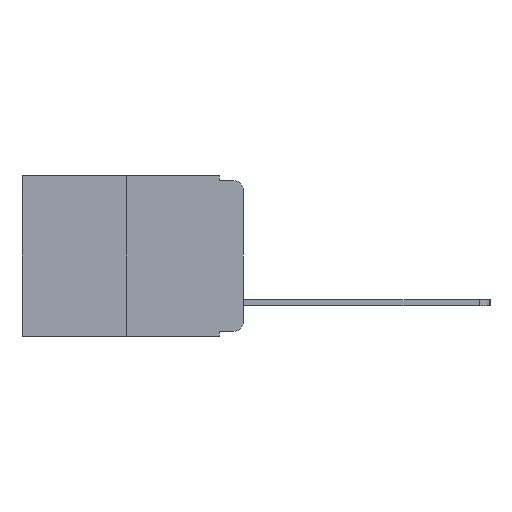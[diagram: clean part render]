
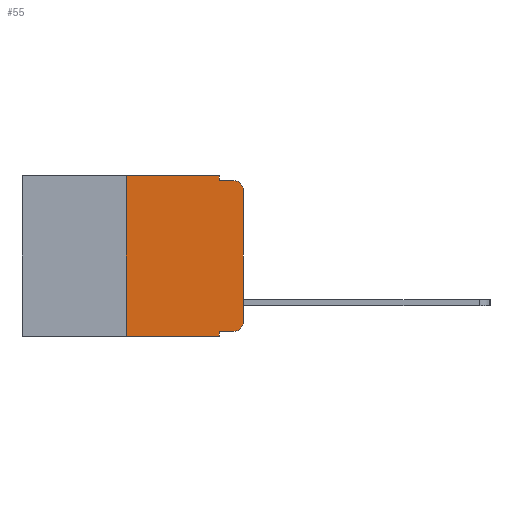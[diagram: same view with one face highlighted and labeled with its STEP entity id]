
A CAD part, left-side view. The second image highlights one B-rep face of the part: STEP entity #55.
In plain terms, the highlighted planar face has unit normal (-1, 0, 0).
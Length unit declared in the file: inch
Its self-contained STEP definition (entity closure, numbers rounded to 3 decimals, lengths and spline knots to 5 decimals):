
#55 = ADVANCED_FACE ( 'NONE', ( #7091 ), #18615, .F. ) ;
#433 = VECTOR ( 'NONE', #20147, 39.37008 ) ;
#586 = VECTOR ( 'NONE', #16774, 39.37008 ) ;
#597 = VERTEX_POINT ( 'NONE', #14116 ) ;
#598 = VERTEX_POINT ( 'NONE', #16816 ) ;
#1123 = ORIENTED_EDGE ( 'NONE', *, *, #10731, .F. ) ;
#1836 = EDGE_LOOP ( 'NONE', ( #14913, #14934, #15651, #18490, #20879, #17882, #7262, #1123, #14017, #13788 ) ) ;
#1862 = VERTEX_POINT ( 'NONE', #4529 ) ;
#2223 = DIRECTION ( 'NONE',  ( -1., 0., 0. ) ) ;
#2350 = CIRCLE ( 'NONE', #5053, 0.02 ) ;
#2389 = LINE ( 'NONE', #4756, #18641 ) ;
#2857 = DIRECTION ( 'NONE',  ( 1., 0., 0. ) ) ;
#3148 = VERTEX_POINT ( 'NONE', #18737 ) ;
#3492 = CARTESIAN_POINT ( 'NONE',  ( 0., 0.25, 0. ) ) ;
#3639 = VERTEX_POINT ( 'NONE', #6182 ) ;
#3965 = EDGE_CURVE ( 'NONE', #8774, #598, #14418, .T. ) ;
#4018 = DIRECTION ( 'NONE',  ( -1., 0., 0. ) ) ;
#4388 = EDGE_CURVE ( 'NONE', #3639, #8774, #10649, .T. ) ;
#4433 = LINE ( 'NONE', #15539, #433 ) ;
#4529 = CARTESIAN_POINT ( 'NONE',  ( 0., 0., -0.03 ) ) ;
#4756 = CARTESIAN_POINT ( 'NONE',  ( 0., 0.051, -0.333 ) ) ;
#5053 = AXIS2_PLACEMENT_3D ( 'NONE', #12225, #2223, #13810 ) ;
#5112 = DIRECTION ( 'NONE',  ( 0., 0., -1. ) ) ;
#5128 = LINE ( 'NONE', #10507, #586 ) ;
#5512 = DIRECTION ( 'NONE',  ( 0., -1., 0. ) ) ;
#5870 = AXIS2_PLACEMENT_3D ( 'NONE', #13924, #4018, #15485 ) ;
#6182 = CARTESIAN_POINT ( 'NONE',  ( 0., 0.051, 0. ) ) ;
#6420 = DIRECTION ( 'NONE',  ( 0., -1., 0. ) ) ;
#7091 = FACE_OUTER_BOUND ( 'NONE', #1836, .T. ) ;
#7262 = ORIENTED_EDGE ( 'NONE', *, *, #19911, .T. ) ;
#7589 = VECTOR ( 'NONE', #18061, 39.37008 ) ;
#7633 = VERTEX_POINT ( 'NONE', #9218 ) ;
#7759 = VECTOR ( 'NONE', #12887, 39.37008 ) ;
#8505 = EDGE_CURVE ( 'NONE', #597, #19544, #2389, .T. ) ;
#8774 = VERTEX_POINT ( 'NONE', #13758 ) ;
#8982 = CARTESIAN_POINT ( 'NONE',  ( 0., 0.051, -0.01 ) ) ;
#9213 = EDGE_CURVE ( 'NONE', #1862, #598, #2350, .T. ) ;
#9218 = CARTESIAN_POINT ( 'NONE',  ( 0., 0.25, -0.343 ) ) ;
#9565 = CARTESIAN_POINT ( 'NONE',  ( 0., 0.473, 0. ) ) ;
#10163 = VECTOR ( 'NONE', #5512, 39.37008 ) ;
#10241 = CARTESIAN_POINT ( 'NONE',  ( 0., 0.051, 0. ) ) ;
#10507 = CARTESIAN_POINT ( 'NONE',  ( 0., 0.473, 0. ) ) ;
#10523 = CARTESIAN_POINT ( 'NONE',  ( 0., 0.02, -0.333 ) ) ;
#10649 = LINE ( 'NONE', #15054, #15355 ) ;
#10731 = EDGE_CURVE ( 'NONE', #597, #19695, #20265, .T. ) ;
#11412 = CARTESIAN_POINT ( 'NONE',  ( 0., 0.25, 0. ) ) ;
#12146 = LINE ( 'NONE', #15963, #7759 ) ;
#12225 = CARTESIAN_POINT ( 'NONE',  ( 0., 0.02, -0.03 ) ) ;
#12887 = DIRECTION ( 'NONE',  ( 0., -1., 0. ) ) ;
#13758 = CARTESIAN_POINT ( 'NONE',  ( 0., 0.051, -0.01 ) ) ;
#13788 = ORIENTED_EDGE ( 'NONE', *, *, #18495, .T. ) ;
#13810 = DIRECTION ( 'NONE',  ( 0., 0., -1. ) ) ;
#13924 = CARTESIAN_POINT ( 'NONE',  ( 0., 0.02, -0.313 ) ) ;
#14003 = CARTESIAN_POINT ( 'NONE',  ( 0., 0.051, -0.343 ) ) ;
#14017 = ORIENTED_EDGE ( 'NONE', *, *, #8505, .T. ) ;
#14116 = CARTESIAN_POINT ( 'NONE',  ( 0., 0.051, -0.333 ) ) ;
#14418 = LINE ( 'NONE', #8982, #10163 ) ;
#14667 = CIRCLE ( 'NONE', #5870, 0.02 ) ;
#14913 = ORIENTED_EDGE ( 'NONE', *, *, #16514, .T. ) ;
#14934 = ORIENTED_EDGE ( 'NONE', *, *, #9213, .T. ) ;
#15054 = CARTESIAN_POINT ( 'NONE',  ( 0., 0.051, 0. ) ) ;
#15216 = VECTOR ( 'NONE', #18025, 39.37008 ) ;
#15355 = VECTOR ( 'NONE', #5112, 39.37008 ) ;
#15485 = DIRECTION ( 'NONE',  ( 0., 0., -1. ) ) ;
#15539 = CARTESIAN_POINT ( 'NONE',  ( 0., 0., 0. ) ) ;
#15651 = ORIENTED_EDGE ( 'NONE', *, *, #3965, .F. ) ;
#15963 = CARTESIAN_POINT ( 'NONE',  ( 0., 0.473, -0.343 ) ) ;
#16398 = EDGE_CURVE ( 'NONE', #7633, #17026, #19322, .T. ) ;
#16514 = EDGE_CURVE ( 'NONE', #3148, #1862, #4433, .T. ) ;
#16774 = DIRECTION ( 'NONE',  ( 0., -1., 0. ) ) ;
#16816 = CARTESIAN_POINT ( 'NONE',  ( 0., 0.02, -0.01 ) ) ;
#17026 = VERTEX_POINT ( 'NONE', #11412 ) ;
#17521 = DIRECTION ( 'NONE',  ( 0., 0., -1. ) ) ;
#17882 = ORIENTED_EDGE ( 'NONE', *, *, #16398, .F. ) ;
#18025 = DIRECTION ( 'NONE',  ( 0., 0., 1. ) ) ;
#18061 = DIRECTION ( 'NONE',  ( 0., 0., -1. ) ) ;
#18289 = AXIS2_PLACEMENT_3D ( 'NONE', #9565, #2857, #17521 ) ;
#18490 = ORIENTED_EDGE ( 'NONE', *, *, #4388, .F. ) ;
#18495 = EDGE_CURVE ( 'NONE', #19544, #3148, #14667, .T. ) ;
#18615 = PLANE ( 'NONE',  #18289 ) ;
#18641 = VECTOR ( 'NONE', #6420, 39.37008 ) ;
#18737 = CARTESIAN_POINT ( 'NONE',  ( 0., 0., -0.313 ) ) ;
#19322 = LINE ( 'NONE', #3492, #15216 ) ;
#19544 = VERTEX_POINT ( 'NONE', #10523 ) ;
#19606 = EDGE_CURVE ( 'NONE', #17026, #3639, #5128, .T. ) ;
#19695 = VERTEX_POINT ( 'NONE', #14003 ) ;
#19911 = EDGE_CURVE ( 'NONE', #7633, #19695, #12146, .T. ) ;
#20147 = DIRECTION ( 'NONE',  ( 0., 0., 1. ) ) ;
#20265 = LINE ( 'NONE', #10241, #7589 ) ;
#20879 = ORIENTED_EDGE ( 'NONE', *, *, #19606, .F. ) ;
